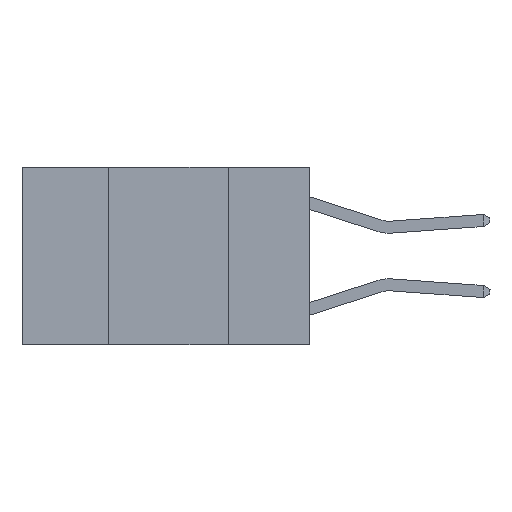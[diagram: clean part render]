
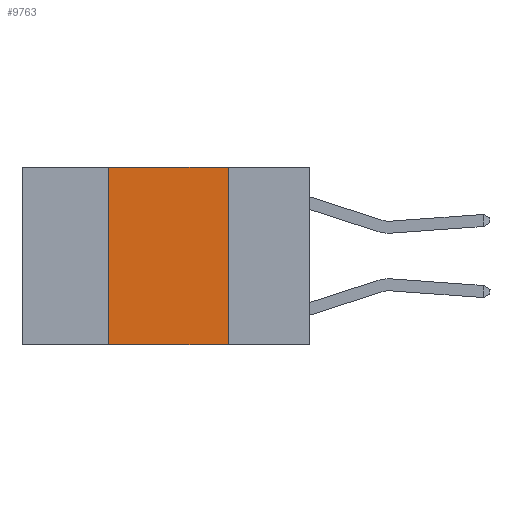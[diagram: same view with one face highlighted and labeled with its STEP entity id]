
A CAD part, left-side view. The second image highlights one B-rep face of the part: STEP entity #9763.
In plain terms, the highlighted planar face has unit normal (-1, 0, 0).
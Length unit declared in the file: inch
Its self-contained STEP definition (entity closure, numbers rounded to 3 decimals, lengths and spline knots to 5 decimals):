
#283 = DIRECTION ( 'NONE',  ( 1., 0., 0. ) ) ;
#630 = DIRECTION ( 'NONE',  ( 0., 0., -1. ) ) ;
#843 = CARTESIAN_POINT ( 'NONE',  ( 0., 0.17, -0.37 ) ) ;
#1177 = VECTOR ( 'NONE', #630, 39.37008 ) ;
#1545 = CARTESIAN_POINT ( 'NONE',  ( 0., 0.6, 0. ) ) ;
#1621 = CARTESIAN_POINT ( 'NONE',  ( 0., 0.6, -0.37 ) ) ;
#2601 = CARTESIAN_POINT ( 'NONE',  ( 0., 0.42, -0.37 ) ) ;
#2950 = VERTEX_POINT ( 'NONE', #2601 ) ;
#2955 = ORIENTED_EDGE ( 'NONE', *, *, #13121, .F. ) ;
#3565 = EDGE_LOOP ( 'NONE', ( #13281, #13724, #2955, #8079 ) ) ;
#3815 = EDGE_CURVE ( 'NONE', #10612, #13696, #15384, .T. ) ;
#4373 = LINE ( 'NONE', #1621, #14940 ) ;
#5773 = PLANE ( 'NONE',  #10952 ) ;
#5940 = CARTESIAN_POINT ( 'NONE',  ( 0., 0.17, 0. ) ) ;
#8079 = ORIENTED_EDGE ( 'NONE', *, *, #9749, .T. ) ;
#8486 = EDGE_CURVE ( 'NONE', #12758, #10612, #14985, .T. ) ;
#9401 = DIRECTION ( 'NONE',  ( 0., 0., 1. ) ) ;
#9749 = EDGE_CURVE ( 'NONE', #2950, #13696, #4373, .T. ) ;
#9763 = ADVANCED_FACE ( 'NONE', ( #11228 ), #5773, .F. ) ;
#9885 = DIRECTION ( 'NONE',  ( 0., 0., -1. ) ) ;
#10429 = VECTOR ( 'NONE', #13931, 39.37008 ) ;
#10612 = VERTEX_POINT ( 'NONE', #14863 ) ;
#10952 = AXIS2_PLACEMENT_3D ( 'NONE', #11180, #283, #9885 ) ;
#11180 = CARTESIAN_POINT ( 'NONE',  ( 0., 0.6, 0. ) ) ;
#11228 = FACE_OUTER_BOUND ( 'NONE', #3565, .T. ) ;
#12604 = DIRECTION ( 'NONE',  ( 0., -1., 0. ) ) ;
#12758 = VERTEX_POINT ( 'NONE', #15154 ) ;
#12842 = LINE ( 'NONE', #17634, #13730 ) ;
#13121 = EDGE_CURVE ( 'NONE', #2950, #12758, #12842, .T. ) ;
#13281 = ORIENTED_EDGE ( 'NONE', *, *, #3815, .F. ) ;
#13696 = VERTEX_POINT ( 'NONE', #843 ) ;
#13724 = ORIENTED_EDGE ( 'NONE', *, *, #8486, .F. ) ;
#13730 = VECTOR ( 'NONE', #9401, 39.37008 ) ;
#13931 = DIRECTION ( 'NONE',  ( 0., -1., 0. ) ) ;
#14863 = CARTESIAN_POINT ( 'NONE',  ( 0., 0.17, 0. ) ) ;
#14940 = VECTOR ( 'NONE', #12604, 39.37008 ) ;
#14985 = LINE ( 'NONE', #1545, #10429 ) ;
#15154 = CARTESIAN_POINT ( 'NONE',  ( 0., 0.42, 0. ) ) ;
#15384 = LINE ( 'NONE', #5940, #1177 ) ;
#17634 = CARTESIAN_POINT ( 'NONE',  ( 0., 0.42, 0. ) ) ;
